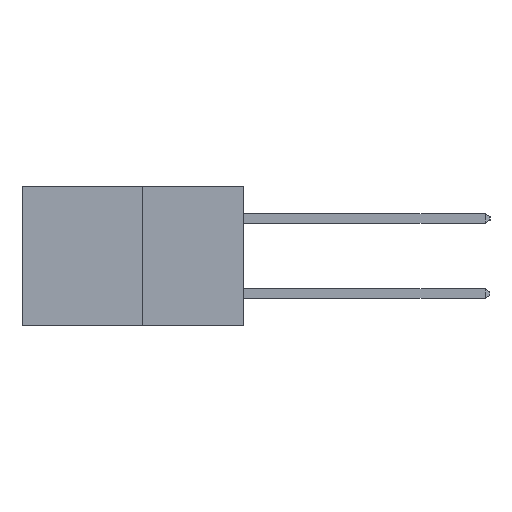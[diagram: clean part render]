
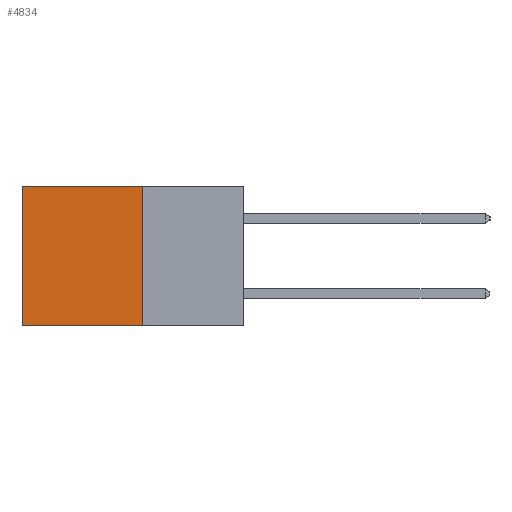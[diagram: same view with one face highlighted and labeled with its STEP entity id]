
A CAD part, left-side view. The second image highlights one B-rep face of the part: STEP entity #4834.
In plain terms, the highlighted planar face has unit normal (-1, 0, 0).
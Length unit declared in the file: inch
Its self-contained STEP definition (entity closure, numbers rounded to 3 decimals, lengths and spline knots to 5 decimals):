
#290 = LINE ( 'NONE', #4054, #12603 ) ;
#404 = EDGE_LOOP ( 'NONE', ( #8638, #6878, #7181, #2178 ) ) ;
#575 = DIRECTION ( 'NONE',  ( 0., 0., -1. ) ) ;
#589 = DIRECTION ( 'NONE',  ( 1., 0., 0. ) ) ;
#629 = PLANE ( 'NONE',  #5790 ) ;
#824 = CARTESIAN_POINT ( 'NONE',  ( 0.277, 0.27, -0.37 ) ) ;
#1453 = VECTOR ( 'NONE', #10366, 39.37008 ) ;
#2104 = FACE_OUTER_BOUND ( 'NONE', #404, .T. ) ;
#2178 = ORIENTED_EDGE ( 'NONE', *, *, #6242, .T. ) ;
#2234 = LINE ( 'NONE', #7451, #14471 ) ;
#3664 = CARTESIAN_POINT ( 'NONE',  ( 0.277, 0.27, 0. ) ) ;
#3817 = VERTEX_POINT ( 'NONE', #11509 ) ;
#4042 = CARTESIAN_POINT ( 'NONE',  ( 0.277, 0.59, 0. ) ) ;
#4054 = CARTESIAN_POINT ( 'NONE',  ( 0.277, 0.59, -0.37 ) ) ;
#4305 = CARTESIAN_POINT ( 'NONE',  ( 0.277, 0.27, -0.37 ) ) ;
#4834 = ADVANCED_FACE ( 'NONE', ( #2104 ), #629, .F. ) ;
#5241 = EDGE_CURVE ( 'NONE', #15013, #3817, #12913, .T. ) ;
#5790 = AXIS2_PLACEMENT_3D ( 'NONE', #824, #589, #575 ) ;
#6242 = EDGE_CURVE ( 'NONE', #14764, #7010, #2234, .T. ) ;
#6878 = ORIENTED_EDGE ( 'NONE', *, *, #5241, .F. ) ;
#7010 = VERTEX_POINT ( 'NONE', #4042 ) ;
#7181 = ORIENTED_EDGE ( 'NONE', *, *, #7232, .F. ) ;
#7232 = EDGE_CURVE ( 'NONE', #14764, #15013, #10941, .T. ) ;
#7451 = CARTESIAN_POINT ( 'NONE',  ( 0.277, 0.27, 0. ) ) ;
#8227 = EDGE_CURVE ( 'NONE', #7010, #3817, #290, .T. ) ;
#8638 = ORIENTED_EDGE ( 'NONE', *, *, #8227, .T. ) ;
#9146 = CARTESIAN_POINT ( 'NONE',  ( 0.277, 0.27, -0.37 ) ) ;
#10081 = VECTOR ( 'NONE', #12637, 39.37008 ) ;
#10366 = DIRECTION ( 'NONE',  ( 0., 0., -1. ) ) ;
#10941 = LINE ( 'NONE', #9146, #1453 ) ;
#11509 = CARTESIAN_POINT ( 'NONE',  ( 0.277, 0.59, -0.37 ) ) ;
#12603 = VECTOR ( 'NONE', #14688, 39.37008 ) ;
#12637 = DIRECTION ( 'NONE',  ( 0., 1., 0. ) ) ;
#12913 = LINE ( 'NONE', #4305, #10081 ) ;
#14471 = VECTOR ( 'NONE', #14500, 39.37008 ) ;
#14500 = DIRECTION ( 'NONE',  ( 0., 1., 0. ) ) ;
#14688 = DIRECTION ( 'NONE',  ( 0., 0., -1. ) ) ;
#14725 = CARTESIAN_POINT ( 'NONE',  ( 0.277, 0.27, -0.37 ) ) ;
#14764 = VERTEX_POINT ( 'NONE', #3664 ) ;
#15013 = VERTEX_POINT ( 'NONE', #14725 ) ;
